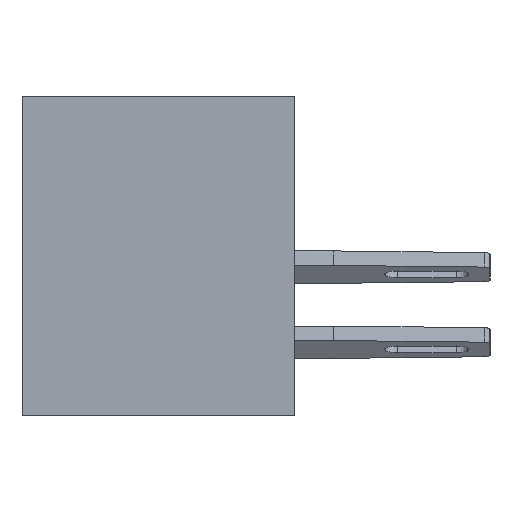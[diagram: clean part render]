
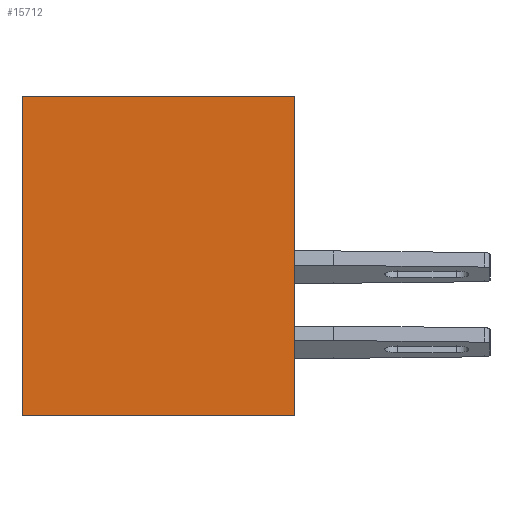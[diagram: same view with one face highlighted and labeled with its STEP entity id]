
A CAD part, left-side view. The second image highlights one B-rep face of the part: STEP entity #15712.
In plain terms, the highlighted planar face has unit normal (-1, 0, 0).
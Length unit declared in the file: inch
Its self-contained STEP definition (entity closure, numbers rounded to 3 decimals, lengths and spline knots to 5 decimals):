
#701 = VECTOR ( 'NONE', #10141, 39.37008 ) ;
#932 = CARTESIAN_POINT ( 'NONE',  ( 0., 0., 0. ) ) ;
#1160 = VECTOR ( 'NONE', #7861, 39.37008 ) ;
#1832 = LINE ( 'NONE', #2750, #701 ) ;
#2750 = CARTESIAN_POINT ( 'NONE',  ( 0., 0.453, 0. ) ) ;
#2888 = CARTESIAN_POINT ( 'NONE',  ( 0., 0.453, 0. ) ) ;
#3235 = CARTESIAN_POINT ( 'NONE',  ( 0., 0.453, 0. ) ) ;
#3801 = LINE ( 'NONE', #11268, #6691 ) ;
#3947 = CARTESIAN_POINT ( 'NONE',  ( 0., 0.453, -0.531 ) ) ;
#4367 = LINE ( 'NONE', #11423, #1160 ) ;
#4689 = ORIENTED_EDGE ( 'NONE', *, *, #9629, .T. ) ;
#4850 = CARTESIAN_POINT ( 'NONE',  ( 0., 0.453, 0. ) ) ;
#5103 = EDGE_CURVE ( 'NONE', #11538, #11211, #1832, .T. ) ;
#5275 = VERTEX_POINT ( 'NONE', #932 ) ;
#5339 = DIRECTION ( 'NONE',  ( 1., 0., 0. ) ) ;
#5564 = ORIENTED_EDGE ( 'NONE', *, *, #15417, .F. ) ;
#5985 = VERTEX_POINT ( 'NONE', #12257 ) ;
#6216 = DIRECTION ( 'NONE',  ( 0., -1., 0. ) ) ;
#6691 = VECTOR ( 'NONE', #6216, 39.37008 ) ;
#6707 = LINE ( 'NONE', #4850, #7261 ) ;
#7057 = EDGE_LOOP ( 'NONE', ( #8961, #5564, #14321, #4689 ) ) ;
#7261 = VECTOR ( 'NONE', #13431, 39.37008 ) ;
#7787 = FACE_OUTER_BOUND ( 'NONE', #7057, .T. ) ;
#7796 = DIRECTION ( 'NONE',  ( 0., 0., -1. ) ) ;
#7861 = DIRECTION ( 'NONE',  ( 0., 0., 1. ) ) ;
#8961 = ORIENTED_EDGE ( 'NONE', *, *, #9869, .T. ) ;
#9629 = EDGE_CURVE ( 'NONE', #11538, #5985, #3801, .T. ) ;
#9869 = EDGE_CURVE ( 'NONE', #5985, #5275, #4367, .T. ) ;
#10141 = DIRECTION ( 'NONE',  ( 0., 0., 1. ) ) ;
#10622 = AXIS2_PLACEMENT_3D ( 'NONE', #2888, #5339, #7796 ) ;
#11211 = VERTEX_POINT ( 'NONE', #3235 ) ;
#11268 = CARTESIAN_POINT ( 'NONE',  ( 0., 0.453, -0.531 ) ) ;
#11423 = CARTESIAN_POINT ( 'NONE',  ( 0., 0., 0. ) ) ;
#11467 = PLANE ( 'NONE',  #10622 ) ;
#11538 = VERTEX_POINT ( 'NONE', #3947 ) ;
#12257 = CARTESIAN_POINT ( 'NONE',  ( 0., 0., -0.531 ) ) ;
#13431 = DIRECTION ( 'NONE',  ( 0., -1., 0. ) ) ;
#14321 = ORIENTED_EDGE ( 'NONE', *, *, #5103, .F. ) ;
#15417 = EDGE_CURVE ( 'NONE', #11211, #5275, #6707, .T. ) ;
#15712 = ADVANCED_FACE ( 'NONE', ( #7787 ), #11467, .F. ) ;
